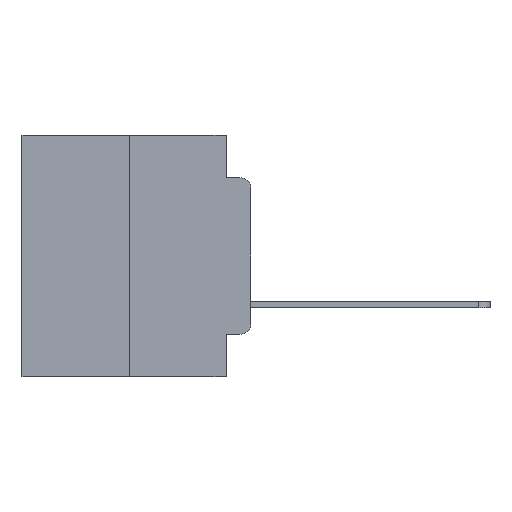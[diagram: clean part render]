
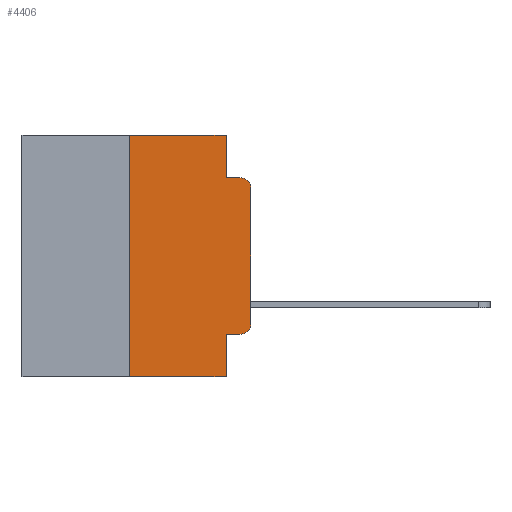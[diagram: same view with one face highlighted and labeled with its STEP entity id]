
A CAD part, left-side view. The second image highlights one B-rep face of the part: STEP entity #4406.
In plain terms, the highlighted planar face has unit normal (-1, 0, 0).
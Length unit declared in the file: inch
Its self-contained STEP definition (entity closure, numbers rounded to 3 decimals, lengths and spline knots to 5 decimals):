
#55 = AXIS2_PLACEMENT_3D ( 'NONE', #21209, #25240, #14688 ) ;
#120 = VERTEX_POINT ( 'NONE', #20823 ) ;
#155 = VERTEX_POINT ( 'NONE', #27103 ) ;
#338 = VECTOR ( 'NONE', #1634, 39.37008 ) ;
#878 = ORIENTED_EDGE ( 'NONE', *, *, #15246, .T. ) ;
#1634 = DIRECTION ( 'NONE',  ( 0., -1., 0. ) ) ;
#1702 = VERTEX_POINT ( 'NONE', #15792 ) ;
#2403 = PLANE ( 'NONE',  #18968 ) ;
#2673 = LINE ( 'NONE', #18552, #338 ) ;
#3201 = ORIENTED_EDGE ( 'NONE', *, *, #22857, .T. ) ;
#3637 = VECTOR ( 'NONE', #25504, 39.37008 ) ;
#4023 = VECTOR ( 'NONE', #12916, 39.37008 ) ;
#4088 = DIRECTION ( 'NONE',  ( 0., 0., -1. ) ) ;
#4406 = ADVANCED_FACE ( 'NONE', ( #14546 ), #2403, .F. ) ;
#4505 = CARTESIAN_POINT ( 'NONE',  ( 0., 0.051, -0.5 ) ) ;
#5118 = CARTESIAN_POINT ( 'NONE',  ( 0., 0.473, 0. ) ) ;
#6132 = DIRECTION ( 'NONE',  ( 0., -1., 0. ) ) ;
#6573 = VECTOR ( 'NONE', #6132, 39.37008 ) ;
#7000 = VERTEX_POINT ( 'NONE', #20473 ) ;
#7468 = CARTESIAN_POINT ( 'NONE',  ( 0., 0.02, -0.3915 ) ) ;
#8711 = ORIENTED_EDGE ( 'NONE', *, *, #26474, .T. ) ;
#8722 = EDGE_CURVE ( 'NONE', #22767, #120, #14249, .T. ) ;
#8778 = LINE ( 'NONE', #22863, #11086 ) ;
#8847 = ORIENTED_EDGE ( 'NONE', *, *, #23606, .T. ) ;
#9322 = DIRECTION ( 'NONE',  ( 0., 0., -1. ) ) ;
#10011 = LINE ( 'NONE', #19153, #15691 ) ;
#10430 = EDGE_LOOP ( 'NONE', ( #3201, #18169, #22464, #26733, #14603, #25103, #8711, #14631, #8847, #878 ) ) ;
#11086 = VECTOR ( 'NONE', #16645, 39.37008 ) ;
#11372 = VECTOR ( 'NONE', #26894, 39.37008 ) ;
#11383 = CIRCLE ( 'NONE', #27441, 0.02 ) ;
#12200 = LINE ( 'NONE', #23147, #6573 ) ;
#12608 = EDGE_CURVE ( 'NONE', #12998, #120, #8778, .T. ) ;
#12916 = DIRECTION ( 'NONE',  ( 0., 0., 1. ) ) ;
#12998 = VERTEX_POINT ( 'NONE', #22012 ) ;
#13927 = CARTESIAN_POINT ( 'NONE',  ( 0., 0.051, -0.4115 ) ) ;
#13949 = CARTESIAN_POINT ( 'NONE',  ( 0., 0.25, -0.5 ) ) ;
#14249 = CIRCLE ( 'NONE', #55, 0.02 ) ;
#14546 = FACE_OUTER_BOUND ( 'NONE', #10430, .T. ) ;
#14603 = ORIENTED_EDGE ( 'NONE', *, *, #21417, .F. ) ;
#14631 = ORIENTED_EDGE ( 'NONE', *, *, #25444, .F. ) ;
#14688 = DIRECTION ( 'NONE',  ( 0., 0., -1. ) ) ;
#15246 = EDGE_CURVE ( 'NONE', #1702, #7000, #11383, .T. ) ;
#15614 = CARTESIAN_POINT ( 'NONE',  ( 0., 0.25, 0. ) ) ;
#15691 = VECTOR ( 'NONE', #4088, 39.37008 ) ;
#15792 = CARTESIAN_POINT ( 'NONE',  ( 0., 0.02, -0.4115 ) ) ;
#16645 = DIRECTION ( 'NONE',  ( 0., -1., 0. ) ) ;
#17139 = CARTESIAN_POINT ( 'NONE',  ( 0., 0.25, 0. ) ) ;
#17930 = VECTOR ( 'NONE', #27475, 39.37008 ) ;
#18065 = LINE ( 'NONE', #5118, #11372 ) ;
#18169 = ORIENTED_EDGE ( 'NONE', *, *, #8722, .T. ) ;
#18257 = VERTEX_POINT ( 'NONE', #15614 ) ;
#18552 = CARTESIAN_POINT ( 'NONE',  ( 0., 0.473, -0.5 ) ) ;
#18968 = AXIS2_PLACEMENT_3D ( 'NONE', #19406, #26046, #9322 ) ;
#19153 = CARTESIAN_POINT ( 'NONE',  ( 0., 0.051, 0. ) ) ;
#19261 = CARTESIAN_POINT ( 'NONE',  ( 0., 0., -0.1085 ) ) ;
#19406 = CARTESIAN_POINT ( 'NONE',  ( 0., 0.473, 0. ) ) ;
#20472 = DIRECTION ( 'NONE',  ( 0., 0., -1. ) ) ;
#20473 = CARTESIAN_POINT ( 'NONE',  ( 0., 0., -0.3915 ) ) ;
#20823 = CARTESIAN_POINT ( 'NONE',  ( 0., 0.02, -0.0885 ) ) ;
#20870 = VERTEX_POINT ( 'NONE', #13949 ) ;
#21209 = CARTESIAN_POINT ( 'NONE',  ( 0., 0.02, -0.1085 ) ) ;
#21417 = EDGE_CURVE ( 'NONE', #18257, #155, #18065, .T. ) ;
#22012 = CARTESIAN_POINT ( 'NONE',  ( 0., 0.051, -0.0885 ) ) ;
#22464 = ORIENTED_EDGE ( 'NONE', *, *, #12608, .F. ) ;
#22497 = EDGE_CURVE ( 'NONE', #20870, #18257, #25667, .T. ) ;
#22767 = VERTEX_POINT ( 'NONE', #19261 ) ;
#22857 = EDGE_CURVE ( 'NONE', #7000, #22767, #24921, .T. ) ;
#22863 = CARTESIAN_POINT ( 'NONE',  ( 0., 0.051, -0.0885 ) ) ;
#23068 = EDGE_CURVE ( 'NONE', #155, #12998, #25228, .T. ) ;
#23147 = CARTESIAN_POINT ( 'NONE',  ( 0., 0.051, -0.4115 ) ) ;
#23341 = CARTESIAN_POINT ( 'NONE',  ( 0., 0., 0. ) ) ;
#23606 = EDGE_CURVE ( 'NONE', #25210, #1702, #12200, .T. ) ;
#24482 = DIRECTION ( 'NONE',  ( -1., 0., 0. ) ) ;
#24921 = LINE ( 'NONE', #23341, #3637 ) ;
#25103 = ORIENTED_EDGE ( 'NONE', *, *, #22497, .F. ) ;
#25210 = VERTEX_POINT ( 'NONE', #13927 ) ;
#25228 = LINE ( 'NONE', #25506, #17930 ) ;
#25240 = DIRECTION ( 'NONE',  ( -1., 0., 0. ) ) ;
#25444 = EDGE_CURVE ( 'NONE', #25210, #26816, #10011, .T. ) ;
#25504 = DIRECTION ( 'NONE',  ( 0., 0., 1. ) ) ;
#25506 = CARTESIAN_POINT ( 'NONE',  ( 0., 0.051, 0. ) ) ;
#25667 = LINE ( 'NONE', #17139, #4023 ) ;
#26046 = DIRECTION ( 'NONE',  ( 1., 0., 0. ) ) ;
#26474 = EDGE_CURVE ( 'NONE', #20870, #26816, #2673, .T. ) ;
#26733 = ORIENTED_EDGE ( 'NONE', *, *, #23068, .F. ) ;
#26816 = VERTEX_POINT ( 'NONE', #4505 ) ;
#26894 = DIRECTION ( 'NONE',  ( 0., -1., 0. ) ) ;
#27103 = CARTESIAN_POINT ( 'NONE',  ( 0., 0.051, 0. ) ) ;
#27441 = AXIS2_PLACEMENT_3D ( 'NONE', #7468, #24482, #20472 ) ;
#27475 = DIRECTION ( 'NONE',  ( 0., 0., -1. ) ) ;
